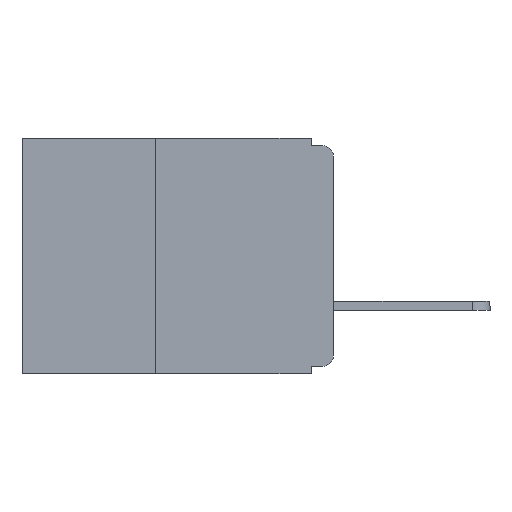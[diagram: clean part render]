
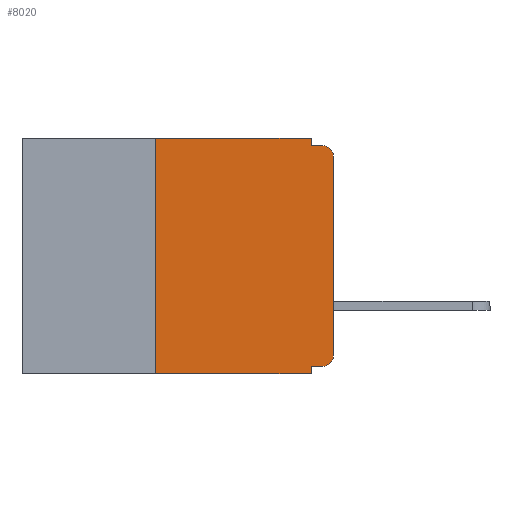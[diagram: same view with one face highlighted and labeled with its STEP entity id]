
A CAD part, left-side view. The second image highlights one B-rep face of the part: STEP entity #8020.
In plain terms, the highlighted planar face has unit normal (-1, 0, 0).
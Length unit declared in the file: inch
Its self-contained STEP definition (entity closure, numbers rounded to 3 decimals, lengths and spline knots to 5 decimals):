
#90 = VECTOR ( 'NONE', #22189, 39.37008 ) ;
#244 = VERTEX_POINT ( 'NONE', #8809 ) ;
#303 = DIRECTION ( 'NONE',  ( 0., 0., -1. ) ) ;
#772 = CARTESIAN_POINT ( 'NONE',  ( 0., 0.031, -0.32 ) ) ;
#1474 = DIRECTION ( 'NONE',  ( 0., 0., -1. ) ) ;
#1706 = LINE ( 'NONE', #4678, #20900 ) ;
#2193 = CARTESIAN_POINT ( 'NONE',  ( 0., 0.25, -0.33 ) ) ;
#2266 = ORIENTED_EDGE ( 'NONE', *, *, #2925, .F. ) ;
#2574 = CARTESIAN_POINT ( 'NONE',  ( 0., 0., -0.01 ) ) ;
#2725 = EDGE_LOOP ( 'NONE', ( #14059, #10145, #2266, #13534, #15759, #3649, #13284, #12440, #8776, #5094 ) ) ;
#2799 = EDGE_CURVE ( 'NONE', #6554, #19899, #5798, .T. ) ;
#2925 = EDGE_CURVE ( 'NONE', #19899, #6202, #21969, .T. ) ;
#3208 = CIRCLE ( 'NONE', #9924, 0.015 ) ;
#3408 = VECTOR ( 'NONE', #10859, 39.37008 ) ;
#3586 = VERTEX_POINT ( 'NONE', #20263 ) ;
#3649 = ORIENTED_EDGE ( 'NONE', *, *, #16249, .F. ) ;
#4031 = DIRECTION ( 'NONE',  ( 0., 0., 1. ) ) ;
#4283 = VERTEX_POINT ( 'NONE', #5359 ) ;
#4666 = VERTEX_POINT ( 'NONE', #2193 ) ;
#4678 = CARTESIAN_POINT ( 'NONE',  ( 0., 0., -0.32 ) ) ;
#5094 = ORIENTED_EDGE ( 'NONE', *, *, #7052, .T. ) ;
#5359 = CARTESIAN_POINT ( 'NONE',  ( 0., 0., -0.305 ) ) ;
#5768 = LINE ( 'NONE', #19071, #10583 ) ;
#5798 = LINE ( 'NONE', #7918, #19655 ) ;
#6202 = VERTEX_POINT ( 'NONE', #10413 ) ;
#6458 = DIRECTION ( 'NONE',  ( -1., 0., 0. ) ) ;
#6554 = VERTEX_POINT ( 'NONE', #14523 ) ;
#7052 = EDGE_CURVE ( 'NONE', #244, #4283, #13538, .T. ) ;
#7595 = VECTOR ( 'NONE', #4031, 39.37008 ) ;
#7918 = CARTESIAN_POINT ( 'NONE',  ( 0., 0.031, 0. ) ) ;
#8020 = ADVANCED_FACE ( 'NONE', ( #14612 ), #21894, .F. ) ;
#8161 = LINE ( 'NONE', #13021, #7595 ) ;
#8189 = VERTEX_POINT ( 'NONE', #772 ) ;
#8351 = VECTOR ( 'NONE', #9017, 39.37008 ) ;
#8776 = ORIENTED_EDGE ( 'NONE', *, *, #15839, .F. ) ;
#8809 = CARTESIAN_POINT ( 'NONE',  ( 0., 0.015, -0.32 ) ) ;
#9017 = DIRECTION ( 'NONE',  ( 0., -1., 0. ) ) ;
#9312 = AXIS2_PLACEMENT_3D ( 'NONE', #16388, #11057, #303 ) ;
#9316 = DIRECTION ( 'NONE',  ( 0., 0., -1. ) ) ;
#9924 = AXIS2_PLACEMENT_3D ( 'NONE', #23096, #12254, #1474 ) ;
#10145 = ORIENTED_EDGE ( 'NONE', *, *, #22145, .T. ) ;
#10413 = CARTESIAN_POINT ( 'NONE',  ( 0., 0.015, -0.01 ) ) ;
#10583 = VECTOR ( 'NONE', #20891, 39.37008 ) ;
#10859 = DIRECTION ( 'NONE',  ( 0., -1., 0. ) ) ;
#11057 = DIRECTION ( 'NONE',  ( 1., 0., 0. ) ) ;
#11376 = CARTESIAN_POINT ( 'NONE',  ( 0., 0.437, 0. ) ) ;
#11935 = EDGE_CURVE ( 'NONE', #3586, #6554, #18087, .T. ) ;
#12254 = DIRECTION ( 'NONE',  ( -1., 0., 0. ) ) ;
#12362 = EDGE_CURVE ( 'NONE', #4666, #13530, #17820, .T. ) ;
#12440 = ORIENTED_EDGE ( 'NONE', *, *, #18595, .F. ) ;
#12882 = VERTEX_POINT ( 'NONE', #16365 ) ;
#13021 = CARTESIAN_POINT ( 'NONE',  ( 0., 0.25, -0.33 ) ) ;
#13284 = ORIENTED_EDGE ( 'NONE', *, *, #12362, .T. ) ;
#13530 = VERTEX_POINT ( 'NONE', #19934 ) ;
#13534 = ORIENTED_EDGE ( 'NONE', *, *, #2799, .F. ) ;
#13538 = CIRCLE ( 'NONE', #20489, 0.015 ) ;
#13549 = EDGE_CURVE ( 'NONE', #4283, #12882, #20609, .T. ) ;
#14059 = ORIENTED_EDGE ( 'NONE', *, *, #13549, .T. ) ;
#14523 = CARTESIAN_POINT ( 'NONE',  ( 0., 0.031, 0. ) ) ;
#14612 = FACE_OUTER_BOUND ( 'NONE', #2725, .T. ) ;
#15201 = VECTOR ( 'NONE', #20008, 39.37008 ) ;
#15759 = ORIENTED_EDGE ( 'NONE', *, *, #11935, .F. ) ;
#15839 = EDGE_CURVE ( 'NONE', #244, #8189, #1706, .T. ) ;
#16249 = EDGE_CURVE ( 'NONE', #4666, #3586, #8161, .T. ) ;
#16365 = CARTESIAN_POINT ( 'NONE',  ( 0., 0., -0.025 ) ) ;
#16388 = CARTESIAN_POINT ( 'NONE',  ( 0., 0.437, 0. ) ) ;
#17249 = CARTESIAN_POINT ( 'NONE',  ( 0., 0.015, -0.305 ) ) ;
#17310 = DIRECTION ( 'NONE',  ( 0., 1., 0. ) ) ;
#17616 = CARTESIAN_POINT ( 'NONE',  ( 0., 0.031, -0.01 ) ) ;
#17820 = LINE ( 'NONE', #21685, #3408 ) ;
#18087 = LINE ( 'NONE', #11376, #90 ) ;
#18178 = CARTESIAN_POINT ( 'NONE',  ( 0., 0., 0. ) ) ;
#18595 = EDGE_CURVE ( 'NONE', #8189, #13530, #5768, .T. ) ;
#19071 = CARTESIAN_POINT ( 'NONE',  ( 0., 0.031, -0.33 ) ) ;
#19076 = DIRECTION ( 'NONE',  ( 0., 0., -1. ) ) ;
#19655 = VECTOR ( 'NONE', #9316, 39.37008 ) ;
#19899 = VERTEX_POINT ( 'NONE', #17616 ) ;
#19934 = CARTESIAN_POINT ( 'NONE',  ( 0., 0.031, -0.33 ) ) ;
#20008 = DIRECTION ( 'NONE',  ( 0., 0., 1. ) ) ;
#20263 = CARTESIAN_POINT ( 'NONE',  ( 0., 0.25, 0. ) ) ;
#20489 = AXIS2_PLACEMENT_3D ( 'NONE', #17249, #6458, #19076 ) ;
#20609 = LINE ( 'NONE', #18178, #15201 ) ;
#20891 = DIRECTION ( 'NONE',  ( 0., 0., -1. ) ) ;
#20900 = VECTOR ( 'NONE', #17310, 39.37008 ) ;
#21685 = CARTESIAN_POINT ( 'NONE',  ( 0., 0.437, -0.33 ) ) ;
#21894 = PLANE ( 'NONE',  #9312 ) ;
#21969 = LINE ( 'NONE', #2574, #8351 ) ;
#22145 = EDGE_CURVE ( 'NONE', #12882, #6202, #3208, .T. ) ;
#22189 = DIRECTION ( 'NONE',  ( 0., -1., 0. ) ) ;
#23096 = CARTESIAN_POINT ( 'NONE',  ( 0., 0.015, -0.025 ) ) ;
